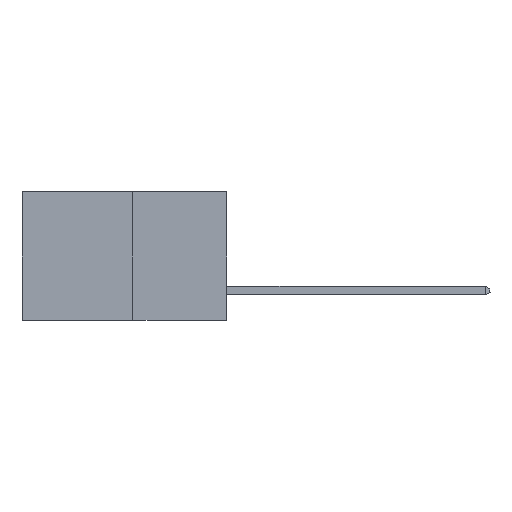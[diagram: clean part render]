
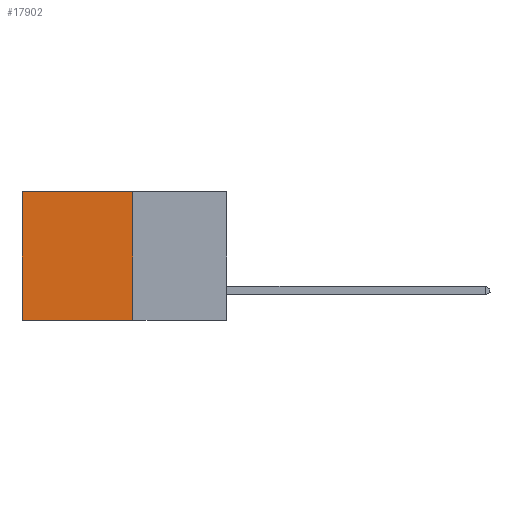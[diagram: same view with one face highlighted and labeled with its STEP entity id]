
A CAD part, left-side view. The second image highlights one B-rep face of the part: STEP entity #17902.
In plain terms, the highlighted planar face has unit normal (-1, 0, 0).
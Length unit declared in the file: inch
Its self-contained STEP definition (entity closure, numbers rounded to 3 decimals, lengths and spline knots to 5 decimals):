
#201 = VECTOR ( 'NONE', #7827, 39.37008 ) ;
#1249 = DIRECTION ( 'NONE',  ( 0., 0., -1. ) ) ;
#1263 = VERTEX_POINT ( 'NONE', #11286 ) ;
#1682 = AXIS2_PLACEMENT_3D ( 'NONE', #5261, #13206, #1249 ) ;
#2888 = FACE_OUTER_BOUND ( 'NONE', #13020, .T. ) ;
#5048 = LINE ( 'NONE', #17562, #20117 ) ;
#5261 = CARTESIAN_POINT ( 'NONE',  ( 0.277, 0.27, -0.37 ) ) ;
#6534 = LINE ( 'NONE', #10296, #7154 ) ;
#6657 = VECTOR ( 'NONE', #15538, 39.37008 ) ;
#7154 = VECTOR ( 'NONE', #24004, 39.37008 ) ;
#7827 = DIRECTION ( 'NONE',  ( 0., 1., 0. ) ) ;
#10186 = CARTESIAN_POINT ( 'NONE',  ( 0.277, 0.27, 0. ) ) ;
#10296 = CARTESIAN_POINT ( 'NONE',  ( 0.277, 0.27, -0.37 ) ) ;
#10732 = ORIENTED_EDGE ( 'NONE', *, *, #14192, .F. ) ;
#11044 = EDGE_CURVE ( 'NONE', #25338, #22112, #15890, .T. ) ;
#11228 = PLANE ( 'NONE',  #1682 ) ;
#11286 = CARTESIAN_POINT ( 'NONE',  ( 0.277, 0.59, -0.37 ) ) ;
#11573 = DIRECTION ( 'NONE',  ( 0., 0., -1. ) ) ;
#11597 = ORIENTED_EDGE ( 'NONE', *, *, #12909, .T. ) ;
#12092 = LINE ( 'NONE', #17601, #201 ) ;
#12909 = EDGE_CURVE ( 'NONE', #22112, #1263, #5048, .T. ) ;
#13020 = EDGE_LOOP ( 'NONE', ( #11597, #10732, #13933, #22764 ) ) ;
#13206 = DIRECTION ( 'NONE',  ( 1., 0., 0. ) ) ;
#13570 = CARTESIAN_POINT ( 'NONE',  ( 0.277, 0.27, 0. ) ) ;
#13933 = ORIENTED_EDGE ( 'NONE', *, *, #21288, .F. ) ;
#14192 = EDGE_CURVE ( 'NONE', #17267, #1263, #12092, .T. ) ;
#15538 = DIRECTION ( 'NONE',  ( 0., 1., 0. ) ) ;
#15890 = LINE ( 'NONE', #13570, #6657 ) ;
#17267 = VERTEX_POINT ( 'NONE', #19233 ) ;
#17562 = CARTESIAN_POINT ( 'NONE',  ( 0.277, 0.59, -0.37 ) ) ;
#17601 = CARTESIAN_POINT ( 'NONE',  ( 0.277, 0.27, -0.37 ) ) ;
#17902 = ADVANCED_FACE ( 'NONE', ( #2888 ), #11228, .F. ) ;
#18593 = CARTESIAN_POINT ( 'NONE',  ( 0.277, 0.59, 0. ) ) ;
#19233 = CARTESIAN_POINT ( 'NONE',  ( 0.277, 0.27, -0.37 ) ) ;
#20117 = VECTOR ( 'NONE', #11573, 39.37008 ) ;
#21288 = EDGE_CURVE ( 'NONE', #25338, #17267, #6534, .T. ) ;
#22112 = VERTEX_POINT ( 'NONE', #18593 ) ;
#22764 = ORIENTED_EDGE ( 'NONE', *, *, #11044, .T. ) ;
#24004 = DIRECTION ( 'NONE',  ( 0., 0., -1. ) ) ;
#25338 = VERTEX_POINT ( 'NONE', #10186 ) ;
